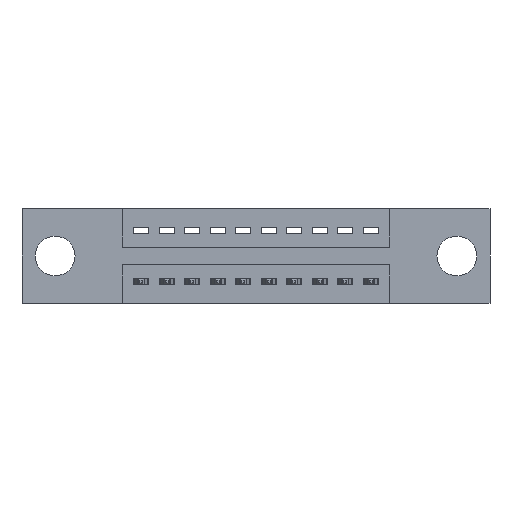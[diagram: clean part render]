
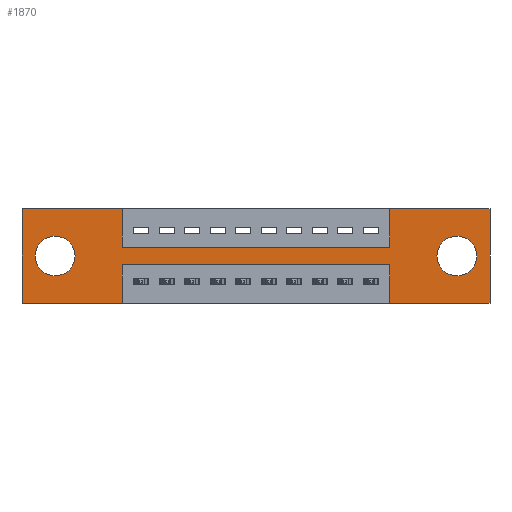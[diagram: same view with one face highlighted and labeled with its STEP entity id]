
A CAD part, front view. The second image highlights one B-rep face of the part: STEP entity #1870.
In plain terms, the highlighted planar face has unit normal (0, -1, 0).
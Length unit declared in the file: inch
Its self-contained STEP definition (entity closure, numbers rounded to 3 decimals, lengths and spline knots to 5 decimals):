
#22 = VERTEX_POINT ( 'NONE', #3446 ) ;
#79 = CIRCLE ( 'NONE', #1244, 0.078 ) ;
#298 = EDGE_CURVE ( 'NONE', #2039, #6872, #8549, .T. ) ;
#370 = CARTESIAN_POINT ( 'NONE',  ( 0., 0., 0. ) ) ;
#435 = ORIENTED_EDGE ( 'NONE', *, *, #7752, .T. ) ;
#510 = CARTESIAN_POINT ( 'NONE',  ( 1.705, 0., -0.107 ) ) ;
#530 = CARTESIAN_POINT ( 'NONE',  ( 1.705, 0., -0.185 ) ) ;
#673 = ORIENTED_EDGE ( 'NONE', *, *, #10888, .T. ) ;
#717 = DIRECTION ( 'NONE',  ( 0., 1., 0. ) ) ;
#763 = EDGE_CURVE ( 'NONE', #3007, #7510, #1120, .T. ) ;
#778 = DIRECTION ( 'NONE',  ( 0., 0., -1. ) ) ;
#943 = EDGE_CURVE ( 'NONE', #7525, #8916, #9544, .T. ) ;
#970 = LINE ( 'NONE', #4878, #10403 ) ;
#1120 = LINE ( 'NONE', #11353, #9252 ) ;
#1244 = AXIS2_PLACEMENT_3D ( 'NONE', #530, #6247, #778 ) ;
#1310 = VERTEX_POINT ( 'NONE', #10987 ) ;
#1322 = ORIENTED_EDGE ( 'NONE', *, *, #9903, .F. ) ;
#1345 = CARTESIAN_POINT ( 'NONE',  ( 0.3925, 0., -0.22 ) ) ;
#1410 = ORIENTED_EDGE ( 'NONE', *, *, #763, .F. ) ;
#1446 = DIRECTION ( 'NONE',  ( 0., 0., 1. ) ) ;
#1577 = DIRECTION ( 'NONE',  ( -1., 0., 0. ) ) ;
#1870 = ADVANCED_FACE ( 'NONE', ( #5650, #11223, #7793 ), #10654, .T. ) ;
#1908 = ORIENTED_EDGE ( 'NONE', *, *, #2604, .F. ) ;
#2037 = CARTESIAN_POINT ( 'NONE',  ( 0.13, 0., -0.185 ) ) ;
#2039 = VERTEX_POINT ( 'NONE', #4476 ) ;
#2135 = DIRECTION ( 'NONE',  ( 0., 0., -1. ) ) ;
#2141 = VERTEX_POINT ( 'NONE', #510 ) ;
#2268 = ORIENTED_EDGE ( 'NONE', *, *, #7679, .F. ) ;
#2574 = DIRECTION ( 'NONE',  ( 0., 1., 0. ) ) ;
#2604 = EDGE_CURVE ( 'NONE', #6872, #3007, #5628, .T. ) ;
#2623 = EDGE_LOOP ( 'NONE', ( #1908, #11700, #11396, #2268, #4115, #8994, #5955, #9271, #8448, #1322, #5314, #1410 ) ) ;
#2818 = DIRECTION ( 'NONE',  ( 0., 0., 1. ) ) ;
#2899 = CARTESIAN_POINT ( 'NONE',  ( 1.4425, 0., 0. ) ) ;
#2963 = CIRCLE ( 'NONE', #5317, 0.078 ) ;
#3007 = VERTEX_POINT ( 'NONE', #5416 ) ;
#3030 = DIRECTION ( 'NONE',  ( -1., 0., 0. ) ) ;
#3143 = EDGE_CURVE ( 'NONE', #8916, #1310, #10038, .T. ) ;
#3168 = VECTOR ( 'NONE', #10597, 39.37008 ) ;
#3321 = EDGE_CURVE ( 'NONE', #10622, #7525, #8233, .T. ) ;
#3379 = VERTEX_POINT ( 'NONE', #11773 ) ;
#3394 = CARTESIAN_POINT ( 'NONE',  ( 1.705, 0., -0.185 ) ) ;
#3397 = EDGE_CURVE ( 'NONE', #2141, #22, #6386, .T. ) ;
#3446 = CARTESIAN_POINT ( 'NONE',  ( 1.705, 0., -0.263 ) ) ;
#3658 = CARTESIAN_POINT ( 'NONE',  ( 1.4425, 0., -0.37 ) ) ;
#3687 = VECTOR ( 'NONE', #4464, 39.37008 ) ;
#4046 = CIRCLE ( 'NONE', #11498, 0.078 ) ;
#4115 = ORIENTED_EDGE ( 'NONE', *, *, #5756, .F. ) ;
#4204 = VERTEX_POINT ( 'NONE', #6356 ) ;
#4269 = LINE ( 'NONE', #11209, #7300 ) ;
#4300 = CARTESIAN_POINT ( 'NONE',  ( 1.4425, 0., 0. ) ) ;
#4336 = DIRECTION ( 'NONE',  ( 0., 0., -1. ) ) ;
#4387 = ORIENTED_EDGE ( 'NONE', *, *, #3397, .T. ) ;
#4464 = DIRECTION ( 'NONE',  ( 0., 0., -1. ) ) ;
#4476 = CARTESIAN_POINT ( 'NONE',  ( 1.4425, 0., -0.22 ) ) ;
#4539 = LINE ( 'NONE', #370, #6572 ) ;
#4878 = CARTESIAN_POINT ( 'NONE',  ( 0., 0., -0.37 ) ) ;
#4901 = CARTESIAN_POINT ( 'NONE',  ( 1.4425, 0., -0.15 ) ) ;
#5136 = DIRECTION ( 'NONE',  ( 0., -1., 0. ) ) ;
#5172 = VECTOR ( 'NONE', #5736, 39.37008 ) ;
#5211 = DIRECTION ( 'NONE',  ( 0., 0., -1. ) ) ;
#5314 = ORIENTED_EDGE ( 'NONE', *, *, #10393, .F. ) ;
#5317 = AXIS2_PLACEMENT_3D ( 'NONE', #2037, #717, #9907 ) ;
#5416 = CARTESIAN_POINT ( 'NONE',  ( 0.3925, 0., -0.37 ) ) ;
#5592 = EDGE_CURVE ( 'NONE', #10319, #2039, #6466, .T. ) ;
#5628 = LINE ( 'NONE', #7750, #3168 ) ;
#5631 = CARTESIAN_POINT ( 'NONE',  ( 0.3925, 0., -0.22 ) ) ;
#5650 = FACE_BOUND ( 'NONE', #9752, .T. ) ;
#5657 = CARTESIAN_POINT ( 'NONE',  ( 0.3925, 0., -0.15 ) ) ;
#5736 = DIRECTION ( 'NONE',  ( 1., 0., 0. ) ) ;
#5756 = EDGE_CURVE ( 'NONE', #1310, #4204, #10012, .T. ) ;
#5926 = EDGE_LOOP ( 'NONE', ( #673, #435 ) ) ;
#5955 = ORIENTED_EDGE ( 'NONE', *, *, #943, .F. ) ;
#6120 = CARTESIAN_POINT ( 'NONE',  ( 0., 0., 0. ) ) ;
#6195 = CARTESIAN_POINT ( 'NONE',  ( 1.835, 0., 0. ) ) ;
#6198 = DIRECTION ( 'NONE',  ( 0., 0., 1. ) ) ;
#6239 = EDGE_CURVE ( 'NONE', #6599, #10622, #4269, .T. ) ;
#6247 = DIRECTION ( 'NONE',  ( 0., 1., 0. ) ) ;
#6356 = CARTESIAN_POINT ( 'NONE',  ( 1.835, 0., -0.37 ) ) ;
#6386 = CIRCLE ( 'NONE', #9737, 0.078 ) ;
#6466 = LINE ( 'NONE', #3658, #10607 ) ;
#6572 = VECTOR ( 'NONE', #10340, 39.37008 ) ;
#6599 = VERTEX_POINT ( 'NONE', #11642 ) ;
#6872 = VERTEX_POINT ( 'NONE', #5631 ) ;
#7060 = DIRECTION ( 'NONE',  ( 1., 0., 0. ) ) ;
#7300 = VECTOR ( 'NONE', #2135, 39.37008 ) ;
#7510 = VERTEX_POINT ( 'NONE', #8089 ) ;
#7525 = VERTEX_POINT ( 'NONE', #4901 ) ;
#7679 = EDGE_CURVE ( 'NONE', #4204, #10319, #970, .T. ) ;
#7702 = CARTESIAN_POINT ( 'NONE',  ( 0.3925, 0., -0.15 ) ) ;
#7750 = CARTESIAN_POINT ( 'NONE',  ( 0.3925, 0., -0.37 ) ) ;
#7752 = EDGE_CURVE ( 'NONE', #11582, #3379, #2963, .T. ) ;
#7793 = FACE_OUTER_BOUND ( 'NONE', #2623, .T. ) ;
#7865 = CARTESIAN_POINT ( 'NONE',  ( 0., 0., -0.37 ) ) ;
#7945 = VECTOR ( 'NONE', #7060, 39.37008 ) ;
#8053 = CARTESIAN_POINT ( 'NONE',  ( 0.13, 0., -0.185 ) ) ;
#8089 = CARTESIAN_POINT ( 'NONE',  ( 0., 0., -0.37 ) ) ;
#8233 = LINE ( 'NONE', #7702, #7945 ) ;
#8419 = CARTESIAN_POINT ( 'NONE',  ( 0., 0., 0. ) ) ;
#8448 = ORIENTED_EDGE ( 'NONE', *, *, #6239, .F. ) ;
#8549 = LINE ( 'NONE', #1345, #9834 ) ;
#8654 = DIRECTION ( 'NONE',  ( -1., 0., 0. ) ) ;
#8717 = AXIS2_PLACEMENT_3D ( 'NONE', #7865, #5136, #5211 ) ;
#8916 = VERTEX_POINT ( 'NONE', #2899 ) ;
#8994 = ORIENTED_EDGE ( 'NONE', *, *, #3143, .F. ) ;
#9250 = EDGE_CURVE ( 'NONE', #22, #2141, #79, .T. ) ;
#9252 = VECTOR ( 'NONE', #3030, 39.37008 ) ;
#9271 = ORIENTED_EDGE ( 'NONE', *, *, #3321, .F. ) ;
#9544 = LINE ( 'NONE', #4300, #10248 ) ;
#9737 = AXIS2_PLACEMENT_3D ( 'NONE', #3394, #9827, #4336 ) ;
#9752 = EDGE_LOOP ( 'NONE', ( #4387, #10675 ) ) ;
#9827 = DIRECTION ( 'NONE',  ( 0., 1., 0. ) ) ;
#9834 = VECTOR ( 'NONE', #8654, 39.37008 ) ;
#9839 = CARTESIAN_POINT ( 'NONE',  ( 0., 0., 0. ) ) ;
#9903 = EDGE_CURVE ( 'NONE', #11049, #6599, #4539, .T. ) ;
#9907 = DIRECTION ( 'NONE',  ( 0., 0., 1. ) ) ;
#10012 = LINE ( 'NONE', #6195, #3687 ) ;
#10038 = LINE ( 'NONE', #8419, #5172 ) ;
#10222 = CARTESIAN_POINT ( 'NONE',  ( 0.13, 0., -0.263 ) ) ;
#10248 = VECTOR ( 'NONE', #6198, 39.37008 ) ;
#10319 = VERTEX_POINT ( 'NONE', #10446 ) ;
#10340 = DIRECTION ( 'NONE',  ( 1., 0., 0. ) ) ;
#10393 = EDGE_CURVE ( 'NONE', #7510, #11049, #11256, .T. ) ;
#10403 = VECTOR ( 'NONE', #1577, 39.37008 ) ;
#10446 = CARTESIAN_POINT ( 'NONE',  ( 1.4425, 0., -0.37 ) ) ;
#10597 = DIRECTION ( 'NONE',  ( 0., 0., -1. ) ) ;
#10607 = VECTOR ( 'NONE', #2818, 39.37008 ) ;
#10622 = VERTEX_POINT ( 'NONE', #5657 ) ;
#10654 = PLANE ( 'NONE',  #8717 ) ;
#10675 = ORIENTED_EDGE ( 'NONE', *, *, #9250, .T. ) ;
#10685 = VECTOR ( 'NONE', #1446, 39.37008 ) ;
#10846 = DIRECTION ( 'NONE',  ( 0., 0., 1. ) ) ;
#10888 = EDGE_CURVE ( 'NONE', #3379, #11582, #4046, .T. ) ;
#10987 = CARTESIAN_POINT ( 'NONE',  ( 1.835, 0., 0. ) ) ;
#11049 = VERTEX_POINT ( 'NONE', #9839 ) ;
#11209 = CARTESIAN_POINT ( 'NONE',  ( 0.3925, 0., 0. ) ) ;
#11223 = FACE_BOUND ( 'NONE', #5926, .T. ) ;
#11256 = LINE ( 'NONE', #6120, #10685 ) ;
#11353 = CARTESIAN_POINT ( 'NONE',  ( 0., 0., -0.37 ) ) ;
#11396 = ORIENTED_EDGE ( 'NONE', *, *, #5592, .F. ) ;
#11498 = AXIS2_PLACEMENT_3D ( 'NONE', #8053, #2574, #10846 ) ;
#11582 = VERTEX_POINT ( 'NONE', #10222 ) ;
#11642 = CARTESIAN_POINT ( 'NONE',  ( 0.3925, 0., 0. ) ) ;
#11700 = ORIENTED_EDGE ( 'NONE', *, *, #298, .F. ) ;
#11773 = CARTESIAN_POINT ( 'NONE',  ( 0.13, 0., -0.107 ) ) ;
